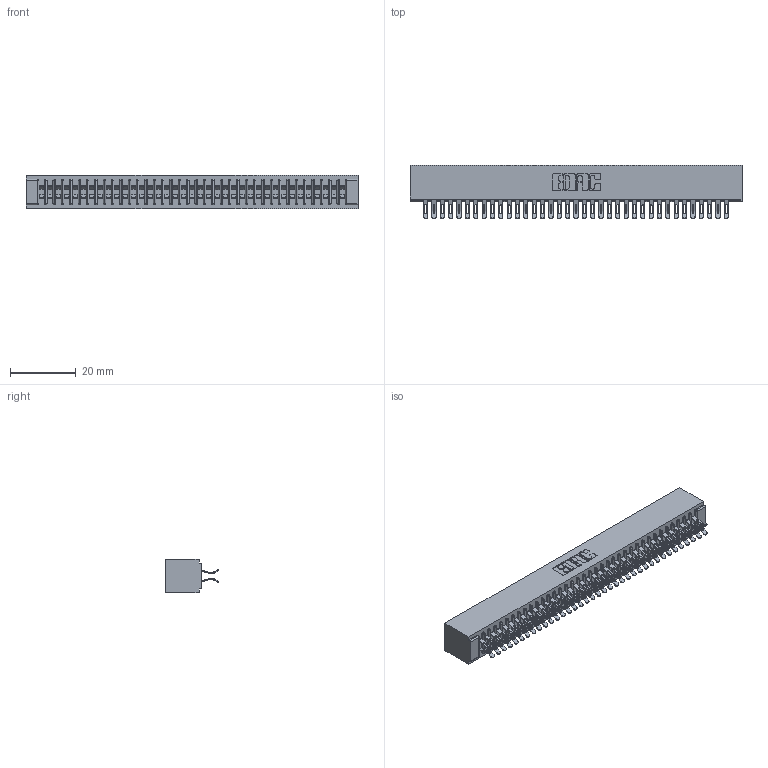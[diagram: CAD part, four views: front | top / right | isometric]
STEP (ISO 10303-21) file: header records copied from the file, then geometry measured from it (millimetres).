
FILE_DESCRIPTION (( 'STEP AP203' ), '1' );
FILE_NAME ('341-074-555-201.STEP', '2018-08-07T20:28:04', ( '' ), ( '' ), 'SwSTEP 2.0', 'SolidWorks 2016', '' );
FILE_SCHEMA (( 'CONFIG_CONTROL_DESIGN' ));
Length unit declared in the file: inch
Products named in the file (3): 341 Part_No Mounting Lugs; 341-292-001_341-292-155; 341-074-555-201
Assembly tree (75 placements, depth 2):
  341-074-555-201
    341 Part_No Mounting Lugs
    341-292-001_341-292-155  x74
Bounding box: 100.97 x 16.31 x 10.16 mm (x, y, z)
Volume: 7781.2 mm3; surface area: 14921 mm2
Topology: 75 solids, 75 shells, 5880 faces, 17571 edges, 11438 vertices
Faces by surface type: plane 3172, cylinder 2560, sphere 76, torus 72
Entity records: 45636 total; most frequent: CARTESIAN_POINT 7601, ORIENTED_EDGE 7542, DIRECTION 7369, EDGE_CURVE 3771, VECTOR 3029, LINE 3029, VERTEX_POINT 2386, AXIS2_PLACEMENT_3D 2170
